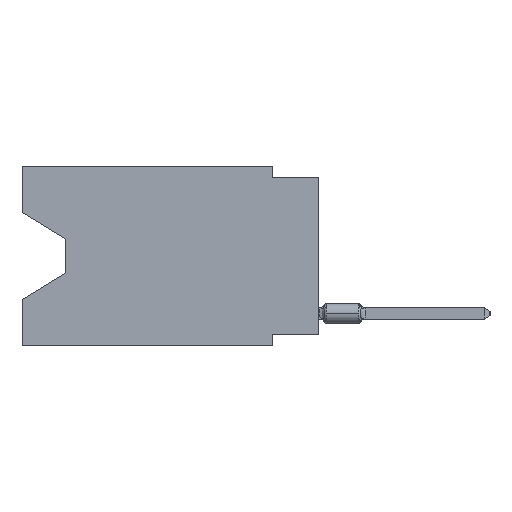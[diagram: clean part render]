
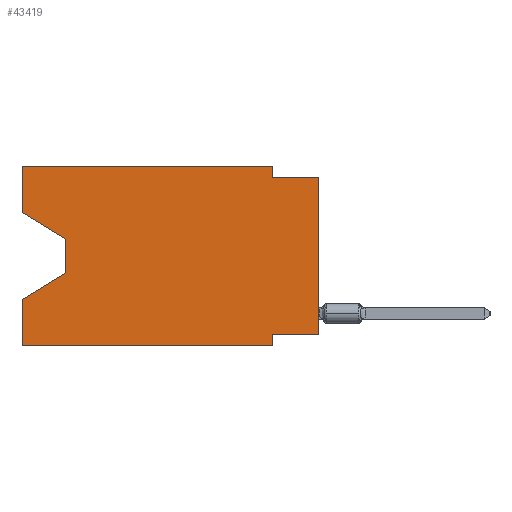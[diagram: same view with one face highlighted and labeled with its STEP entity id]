
A CAD part, left-side view. The second image highlights one B-rep face of the part: STEP entity #43419.
In plain terms, the highlighted planar face has unit normal (-1, 0, 0).
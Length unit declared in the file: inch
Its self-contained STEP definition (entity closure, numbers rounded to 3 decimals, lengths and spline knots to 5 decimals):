
#70 = CARTESIAN_POINT ( 'NONE',  ( 0., 0.645, 0. ) ) ;
#144 = EDGE_CURVE ( 'NONE', #12741, #44357, #48538, .T. ) ;
#1546 = ORIENTED_EDGE ( 'NONE', *, *, #37811, .T. ) ;
#1549 = VECTOR ( 'NONE', #64535, 39.37008 ) ;
#3386 = DIRECTION ( 'NONE',  ( 0., 0.855, -0.519 ) ) ;
#4784 = VECTOR ( 'NONE', #3386, 39.37008 ) ;
#5830 = CARTESIAN_POINT ( 'NONE',  ( 0., 0.645, -0.10025 ) ) ;
#5879 = DIRECTION ( 'NONE',  ( 0., 0., 1. ) ) ;
#5939 = VERTEX_POINT ( 'NONE', #11572 ) ;
#6053 = VERTEX_POINT ( 'NONE', #38787 ) ;
#6285 = CARTESIAN_POINT ( 'NONE',  ( 0., 0.645, -0.10025 ) ) ;
#8620 = CARTESIAN_POINT ( 'NONE',  ( 0., 0.55, -0.232 ) ) ;
#9141 = ORIENTED_EDGE ( 'NONE', *, *, #65539, .F. ) ;
#9219 = CARTESIAN_POINT ( 'NONE',  ( 0., 0.1, -0.39 ) ) ;
#11272 = VECTOR ( 'NONE', #30158, 39.37008 ) ;
#11572 = CARTESIAN_POINT ( 'NONE',  ( 0., 0.1, -0.365 ) ) ;
#11631 = VERTEX_POINT ( 'NONE', #5830 ) ;
#11867 = LINE ( 'NONE', #6285, #1549 ) ;
#12205 = VERTEX_POINT ( 'NONE', #24009 ) ;
#12642 = CARTESIAN_POINT ( 'NONE',  ( 0., 0.1, 0. ) ) ;
#12669 = CARTESIAN_POINT ( 'NONE',  ( 0., 0.55, -0.232 ) ) ;
#12741 = VERTEX_POINT ( 'NONE', #70 ) ;
#15022 = LINE ( 'NONE', #41878, #63029 ) ;
#15148 = EDGE_CURVE ( 'NONE', #38854, #62869, #33306, .T. ) ;
#16480 = EDGE_CURVE ( 'NONE', #56776, #62869, #56400, .T. ) ;
#17621 = CARTESIAN_POINT ( 'NONE',  ( 0., 0.645, -0.39 ) ) ;
#17953 = CARTESIAN_POINT ( 'NONE',  ( 0., 0.645, 0. ) ) ;
#18257 = LINE ( 'NONE', #28718, #52227 ) ;
#20959 = DIRECTION ( 'NONE',  ( 1., 0., 0. ) ) ;
#23409 = LINE ( 'NONE', #61358, #49176 ) ;
#24009 = CARTESIAN_POINT ( 'NONE',  ( 0., 0.1, -0.39 ) ) ;
#24223 = ORIENTED_EDGE ( 'NONE', *, *, #45287, .T. ) ;
#24224 = EDGE_LOOP ( 'NONE', ( #27713, #24223, #41977, #65849, #47217, #28559, #47284, #1546, #9141, #38122, #57378, #49697 ) ) ;
#25142 = DIRECTION ( 'NONE',  ( 0., 0., -1. ) ) ;
#25199 = EDGE_CURVE ( 'NONE', #38854, #12205, #18257, .T. ) ;
#25402 = VECTOR ( 'NONE', #66091, 39.37008 ) ;
#27145 = LINE ( 'NONE', #64457, #64279 ) ;
#27713 = ORIENTED_EDGE ( 'NONE', *, *, #39594, .T. ) ;
#28559 = ORIENTED_EDGE ( 'NONE', *, *, #33279, .F. ) ;
#28718 = CARTESIAN_POINT ( 'NONE',  ( 0., 0.645, -0.39 ) ) ;
#29146 = VERTEX_POINT ( 'NONE', #36617 ) ;
#29685 = PLANE ( 'NONE',  #60742 ) ;
#30158 = DIRECTION ( 'NONE',  ( 0., -1., 0. ) ) ;
#33279 = EDGE_CURVE ( 'NONE', #5939, #12205, #35754, .T. ) ;
#33306 = LINE ( 'NONE', #17953, #33822 ) ;
#33822 = VECTOR ( 'NONE', #59105, 39.37008 ) ;
#34933 = FACE_OUTER_BOUND ( 'NONE', #24224, .T. ) ;
#35754 = LINE ( 'NONE', #9219, #62445 ) ;
#36617 = CARTESIAN_POINT ( 'NONE',  ( 0., 0., -0.365 ) ) ;
#37068 = VERTEX_POINT ( 'NONE', #38652 ) ;
#37442 = CARTESIAN_POINT ( 'NONE',  ( 0., 0.55, -0.158 ) ) ;
#37811 = EDGE_CURVE ( 'NONE', #29146, #37068, #38401, .T. ) ;
#38122 = ORIENTED_EDGE ( 'NONE', *, *, #43536, .F. ) ;
#38401 = LINE ( 'NONE', #59665, #43949 ) ;
#38652 = CARTESIAN_POINT ( 'NONE',  ( 0., 0., -0.025 ) ) ;
#38787 = CARTESIAN_POINT ( 'NONE',  ( 0., 0.1, -0.025 ) ) ;
#38854 = VERTEX_POINT ( 'NONE', #17621 ) ;
#39594 = EDGE_CURVE ( 'NONE', #11631, #52724, #11867, .T. ) ;
#41878 = CARTESIAN_POINT ( 'NONE',  ( 0., 0.1, 0. ) ) ;
#41977 = ORIENTED_EDGE ( 'NONE', *, *, #16480, .T. ) ;
#43310 = DIRECTION ( 'NONE',  ( 0., 0., 1. ) ) ;
#43419 = ADVANCED_FACE ( 'NONE', ( #34933 ), #29685, .F. ) ;
#43536 = EDGE_CURVE ( 'NONE', #44357, #6053, #15022, .T. ) ;
#43949 = VECTOR ( 'NONE', #43310, 39.37008 ) ;
#44357 = VERTEX_POINT ( 'NONE', #12642 ) ;
#44580 = LINE ( 'NONE', #61603, #58755 ) ;
#45111 = EDGE_CURVE ( 'NONE', #11631, #12741, #27145, .T. ) ;
#45287 = EDGE_CURVE ( 'NONE', #52724, #56776, #44580, .T. ) ;
#45767 = EDGE_CURVE ( 'NONE', #29146, #5939, #55290, .T. ) ;
#47217 = ORIENTED_EDGE ( 'NONE', *, *, #25199, .T. ) ;
#47284 = ORIENTED_EDGE ( 'NONE', *, *, #45767, .F. ) ;
#48199 = CARTESIAN_POINT ( 'NONE',  ( 0., 0.645, 0. ) ) ;
#48538 = LINE ( 'NONE', #48199, #11272 ) ;
#49176 = VECTOR ( 'NONE', #62041, 39.37008 ) ;
#49697 = ORIENTED_EDGE ( 'NONE', *, *, #45111, .F. ) ;
#50404 = CARTESIAN_POINT ( 'NONE',  ( 0., 0., -0.365 ) ) ;
#52227 = VECTOR ( 'NONE', #58810, 39.37008 ) ;
#52724 = VERTEX_POINT ( 'NONE', #37442 ) ;
#53034 = CARTESIAN_POINT ( 'NONE',  ( 0., 0.645, 0. ) ) ;
#55290 = LINE ( 'NONE', #50404, #25402 ) ;
#55375 = DIRECTION ( 'NONE',  ( 0., 0., -1. ) ) ;
#55650 = DIRECTION ( 'NONE',  ( 0., 0., -1. ) ) ;
#56400 = LINE ( 'NONE', #8620, #4784 ) ;
#56776 = VERTEX_POINT ( 'NONE', #12669 ) ;
#57378 = ORIENTED_EDGE ( 'NONE', *, *, #144, .F. ) ;
#58755 = VECTOR ( 'NONE', #55375, 39.37008 ) ;
#58810 = DIRECTION ( 'NONE',  ( 0., -1., 0. ) ) ;
#59105 = DIRECTION ( 'NONE',  ( 0., 0., 1. ) ) ;
#59665 = CARTESIAN_POINT ( 'NONE',  ( 0., 0., 0. ) ) ;
#60742 = AXIS2_PLACEMENT_3D ( 'NONE', #53034, #20959, #25142 ) ;
#61358 = CARTESIAN_POINT ( 'NONE',  ( 0., 0., -0.025 ) ) ;
#61603 = CARTESIAN_POINT ( 'NONE',  ( 0., 0.55, -0.158 ) ) ;
#62041 = DIRECTION ( 'NONE',  ( 0., -1., 0. ) ) ;
#62445 = VECTOR ( 'NONE', #55650, 39.37008 ) ;
#62869 = VERTEX_POINT ( 'NONE', #65813 ) ;
#63029 = VECTOR ( 'NONE', #64528, 39.37008 ) ;
#64279 = VECTOR ( 'NONE', #5879, 39.37008 ) ;
#64457 = CARTESIAN_POINT ( 'NONE',  ( 0., 0.645, 0. ) ) ;
#64528 = DIRECTION ( 'NONE',  ( 0., 0., -1. ) ) ;
#64535 = DIRECTION ( 'NONE',  ( 0., -0.855, -0.519 ) ) ;
#65539 = EDGE_CURVE ( 'NONE', #6053, #37068, #23409, .T. ) ;
#65813 = CARTESIAN_POINT ( 'NONE',  ( 0., 0.645, -0.28975 ) ) ;
#65849 = ORIENTED_EDGE ( 'NONE', *, *, #15148, .F. ) ;
#66091 = DIRECTION ( 'NONE',  ( 0., 1., 0. ) ) ;
